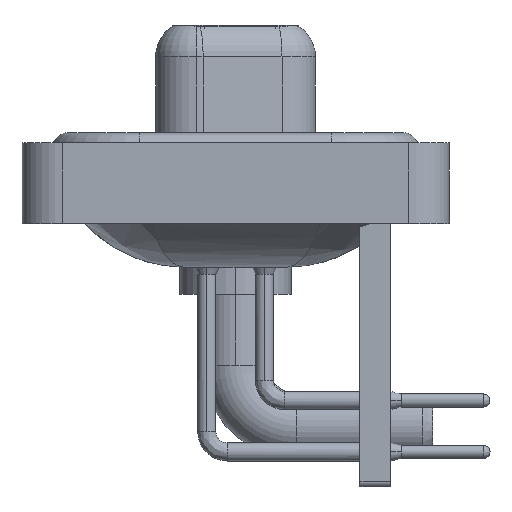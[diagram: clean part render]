
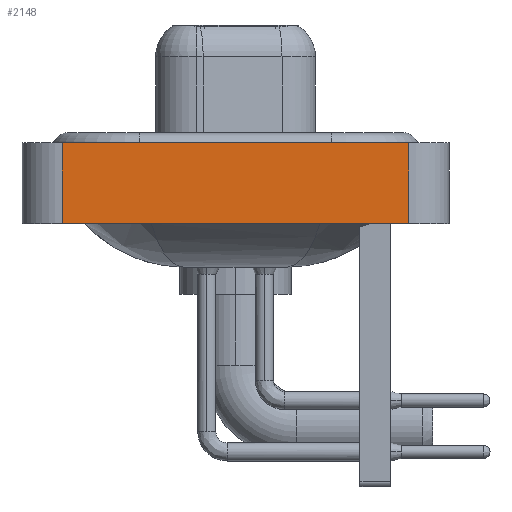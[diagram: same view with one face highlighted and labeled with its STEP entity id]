
A CAD part, left-side view. The second image highlights one B-rep face of the part: STEP entity #2148.
In plain terms, the highlighted planar face has unit normal (-1, 0, 0).
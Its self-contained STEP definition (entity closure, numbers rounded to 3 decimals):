
#792 = DIRECTION ( 'NONE',  ( 0., 0., 1. ) ) ;
#1097 = CARTESIAN_POINT ( 'NONE',  ( -7.25, -8.55, 0.4 ) ) ;
#1283 = LINE ( 'NONE', #7575, #9945 ) ;
#1912 = VECTOR ( 'NONE', #792, 1000. ) ;
#2084 = LINE ( 'NONE', #13060, #1912 ) ;
#2148 = ADVANCED_FACE ( 'NONE', ( #3779 ), #2311, .T. ) ;
#2311 = PLANE ( 'NONE',  #17182 ) ;
#3653 = CARTESIAN_POINT ( 'NONE',  ( -7.25, 8.55, 0.4 ) ) ;
#3779 = FACE_OUTER_BOUND ( 'NONE', #19119, .T. ) ;
#4536 = VECTOR ( 'NONE', #18962, 1000. ) ;
#5721 = ORIENTED_EDGE ( 'NONE', *, *, #12249, .T. ) ;
#5880 = CARTESIAN_POINT ( 'NONE',  ( -7.25, 8.55, -3.6 ) ) ;
#7131 = DIRECTION ( 'NONE',  ( -1., 0., 0. ) ) ;
#7575 = CARTESIAN_POINT ( 'NONE',  ( -7.25, -8.55, -3.6 ) ) ;
#9603 = ORIENTED_EDGE ( 'NONE', *, *, #16834, .F. ) ;
#9833 = EDGE_CURVE ( 'NONE', #14018, #18072, #11081, .T. ) ;
#9945 = VECTOR ( 'NONE', #20416, 1000. ) ;
#10168 = EDGE_CURVE ( 'NONE', #13261, #11898, #1283, .T. ) ;
#10236 = ORIENTED_EDGE ( 'NONE', *, *, #10168, .T. ) ;
#11081 = LINE ( 'NONE', #18855, #4536 ) ;
#11886 = VECTOR ( 'NONE', #19220, 1000. ) ;
#11898 = VERTEX_POINT ( 'NONE', #18402 ) ;
#12249 = EDGE_CURVE ( 'NONE', #11898, #18072, #2084, .T. ) ;
#13060 = CARTESIAN_POINT ( 'NONE',  ( -7.25, -8.55, -3.6 ) ) ;
#13261 = VERTEX_POINT ( 'NONE', #5880 ) ;
#13554 = DIRECTION ( 'NONE',  ( 0., 0., 1. ) ) ;
#14018 = VERTEX_POINT ( 'NONE', #3653 ) ;
#15131 = CARTESIAN_POINT ( 'NONE',  ( -7.25, -8.55, -3.6 ) ) ;
#16834 = EDGE_CURVE ( 'NONE', #13261, #14018, #19120, .T. ) ;
#17182 = AXIS2_PLACEMENT_3D ( 'NONE', #15131, #7131, #13554 ) ;
#17630 = CARTESIAN_POINT ( 'NONE',  ( -7.25, 8.55, -3.6 ) ) ;
#18072 = VERTEX_POINT ( 'NONE', #1097 ) ;
#18402 = CARTESIAN_POINT ( 'NONE',  ( -7.25, -8.55, -3.6 ) ) ;
#18855 = CARTESIAN_POINT ( 'NONE',  ( -7.25, -8.55, 0.4 ) ) ;
#18962 = DIRECTION ( 'NONE',  ( 0., -1., 0. ) ) ;
#19093 = ORIENTED_EDGE ( 'NONE', *, *, #9833, .F. ) ;
#19119 = EDGE_LOOP ( 'NONE', ( #5721, #19093, #9603, #10236 ) ) ;
#19120 = LINE ( 'NONE', #17630, #11886 ) ;
#19220 = DIRECTION ( 'NONE',  ( 0., 0., 1. ) ) ;
#20416 = DIRECTION ( 'NONE',  ( 0., -1., 0. ) ) ;
